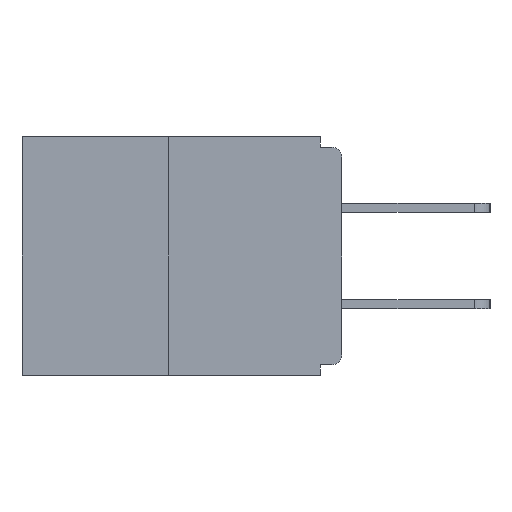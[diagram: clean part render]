
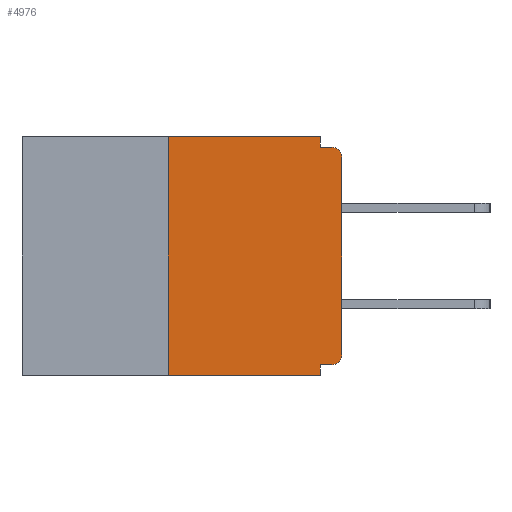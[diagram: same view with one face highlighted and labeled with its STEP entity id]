
A CAD part, left-side view. The second image highlights one B-rep face of the part: STEP entity #4976.
In plain terms, the highlighted planar face has unit normal (-1, 0, 0).
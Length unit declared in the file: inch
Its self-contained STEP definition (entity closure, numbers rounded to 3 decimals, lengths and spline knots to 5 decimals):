
#31 = EDGE_CURVE ( 'NONE', #18143, #26594, #9103, .T. ) ;
#90 = EDGE_CURVE ( 'NONE', #26594, #7525, #13710, .T. ) ;
#605 = AXIS2_PLACEMENT_3D ( 'NONE', #1135, #11697, #5439 ) ;
#971 = LINE ( 'NONE', #27043, #14540 ) ;
#1135 = CARTESIAN_POINT ( 'NONE',  ( 0., 0.015, -0.03 ) ) ;
#1217 = CARTESIAN_POINT ( 'NONE',  ( 0., 0.46, -0.343 ) ) ;
#1404 = ORIENTED_EDGE ( 'NONE', *, *, #26689, .T. ) ;
#2222 = CARTESIAN_POINT ( 'NONE',  ( 0., 0.015, -0.015 ) ) ;
#2550 = EDGE_CURVE ( 'NONE', #18143, #7772, #5038, .T. ) ;
#2584 = DIRECTION ( 'NONE',  ( 0., -1., 0. ) ) ;
#3198 = EDGE_CURVE ( 'NONE', #11646, #19144, #18828, .T. ) ;
#3662 = LINE ( 'NONE', #16313, #14893 ) ;
#3690 = DIRECTION ( 'NONE',  ( 0., 0., 1. ) ) ;
#4295 = CARTESIAN_POINT ( 'NONE',  ( 0., 0.25, -0.343 ) ) ;
#4530 = CARTESIAN_POINT ( 'NONE',  ( 0., 0., -0.03 ) ) ;
#4556 = ORIENTED_EDGE ( 'NONE', *, *, #24536, .T. ) ;
#4976 = ADVANCED_FACE ( 'NONE', ( #19230 ), #17093, .F. ) ;
#5038 = CIRCLE ( 'NONE', #27012, 0.015 ) ;
#5095 = VERTEX_POINT ( 'NONE', #22793 ) ;
#5439 = DIRECTION ( 'NONE',  ( 0., 0., -1. ) ) ;
#5881 = CARTESIAN_POINT ( 'NONE',  ( 0., 0.031, 0. ) ) ;
#6018 = DIRECTION ( 'NONE',  ( 0., 0., 1. ) ) ;
#6752 = LINE ( 'NONE', #5881, #17272 ) ;
#7511 = CIRCLE ( 'NONE', #605, 0.015 ) ;
#7525 = VERTEX_POINT ( 'NONE', #13247 ) ;
#7681 = EDGE_LOOP ( 'NONE', ( #19044, #13883, #1404, #14163, #9592, #15744, #4556, #9803, #15770, #14774 ) ) ;
#7722 = LINE ( 'NONE', #12929, #23861 ) ;
#7772 = VERTEX_POINT ( 'NONE', #14413 ) ;
#7925 = DIRECTION ( 'NONE',  ( 0., 0., -1. ) ) ;
#8393 = CARTESIAN_POINT ( 'NONE',  ( 0., 0.031, -0.343 ) ) ;
#9103 = LINE ( 'NONE', #14466, #15397 ) ;
#9592 = ORIENTED_EDGE ( 'NONE', *, *, #31, .F. ) ;
#9803 = ORIENTED_EDGE ( 'NONE', *, *, #20146, .T. ) ;
#10143 = DIRECTION ( 'NONE',  ( 0., 1., 0. ) ) ;
#11646 = VERTEX_POINT ( 'NONE', #24888 ) ;
#11697 = DIRECTION ( 'NONE',  ( -1., 0., 0. ) ) ;
#12929 = CARTESIAN_POINT ( 'NONE',  ( 0., 0., 0. ) ) ;
#13247 = CARTESIAN_POINT ( 'NONE',  ( 0., 0.031, -0.343 ) ) ;
#13315 = AXIS2_PLACEMENT_3D ( 'NONE', #15324, #21396, #23334 ) ;
#13623 = CARTESIAN_POINT ( 'NONE',  ( 0., 0.25, 0. ) ) ;
#13710 = LINE ( 'NONE', #8393, #18666 ) ;
#13883 = ORIENTED_EDGE ( 'NONE', *, *, #18235, .F. ) ;
#14163 = ORIENTED_EDGE ( 'NONE', *, *, #90, .F. ) ;
#14176 = VECTOR ( 'NONE', #16964, 39.37008 ) ;
#14413 = CARTESIAN_POINT ( 'NONE',  ( 0., 0., -0.313 ) ) ;
#14466 = CARTESIAN_POINT ( 'NONE',  ( 0., 0., -0.328 ) ) ;
#14540 = VECTOR ( 'NONE', #2584, 39.37008 ) ;
#14774 = ORIENTED_EDGE ( 'NONE', *, *, #15347, .F. ) ;
#14893 = VECTOR ( 'NONE', #3690, 39.37008 ) ;
#15324 = CARTESIAN_POINT ( 'NONE',  ( 0., 0.46, 0. ) ) ;
#15347 = EDGE_CURVE ( 'NONE', #5095, #11646, #6752, .T. ) ;
#15397 = VECTOR ( 'NONE', #10143, 39.37008 ) ;
#15744 = ORIENTED_EDGE ( 'NONE', *, *, #2550, .T. ) ;
#15770 = ORIENTED_EDGE ( 'NONE', *, *, #3198, .F. ) ;
#15941 = CARTESIAN_POINT ( 'NONE',  ( 0., 0.015, -0.328 ) ) ;
#16313 = CARTESIAN_POINT ( 'NONE',  ( 0., 0.25, 0. ) ) ;
#16480 = EDGE_CURVE ( 'NONE', #21625, #5095, #971, .T. ) ;
#16964 = DIRECTION ( 'NONE',  ( 0., -1., 0. ) ) ;
#17093 = PLANE ( 'NONE',  #13315 ) ;
#17272 = VECTOR ( 'NONE', #18227, 39.37008 ) ;
#17790 = VECTOR ( 'NONE', #22819, 39.37008 ) ;
#18143 = VERTEX_POINT ( 'NONE', #15941 ) ;
#18227 = DIRECTION ( 'NONE',  ( 0., 0., -1. ) ) ;
#18235 = EDGE_CURVE ( 'NONE', #20836, #21625, #3662, .T. ) ;
#18666 = VECTOR ( 'NONE', #18795, 39.37008 ) ;
#18795 = DIRECTION ( 'NONE',  ( 0., 0., -1. ) ) ;
#18828 = LINE ( 'NONE', #21000, #14176 ) ;
#19044 = ORIENTED_EDGE ( 'NONE', *, *, #16480, .F. ) ;
#19144 = VERTEX_POINT ( 'NONE', #2222 ) ;
#19230 = FACE_OUTER_BOUND ( 'NONE', #7681, .T. ) ;
#19625 = VERTEX_POINT ( 'NONE', #4530 ) ;
#20146 = EDGE_CURVE ( 'NONE', #19625, #19144, #7511, .T. ) ;
#20836 = VERTEX_POINT ( 'NONE', #4295 ) ;
#21000 = CARTESIAN_POINT ( 'NONE',  ( 0., 0., -0.015 ) ) ;
#21396 = DIRECTION ( 'NONE',  ( 1., 0., 0. ) ) ;
#21625 = VERTEX_POINT ( 'NONE', #13623 ) ;
#22665 = CARTESIAN_POINT ( 'NONE',  ( 0., 0.015, -0.313 ) ) ;
#22793 = CARTESIAN_POINT ( 'NONE',  ( 0., 0.031, 0. ) ) ;
#22819 = DIRECTION ( 'NONE',  ( 0., -1., 0. ) ) ;
#23334 = DIRECTION ( 'NONE',  ( 0., 0., -1. ) ) ;
#23861 = VECTOR ( 'NONE', #6018, 39.37008 ) ;
#24536 = EDGE_CURVE ( 'NONE', #7772, #19625, #7722, .T. ) ;
#24868 = DIRECTION ( 'NONE',  ( -1., 0., 0. ) ) ;
#24888 = CARTESIAN_POINT ( 'NONE',  ( 0., 0.031, -0.015 ) ) ;
#25391 = LINE ( 'NONE', #1217, #17790 ) ;
#26050 = CARTESIAN_POINT ( 'NONE',  ( 0., 0.031, -0.328 ) ) ;
#26594 = VERTEX_POINT ( 'NONE', #26050 ) ;
#26689 = EDGE_CURVE ( 'NONE', #20836, #7525, #25391, .T. ) ;
#27012 = AXIS2_PLACEMENT_3D ( 'NONE', #22665, #24868, #7925 ) ;
#27043 = CARTESIAN_POINT ( 'NONE',  ( 0., 0.46, 0. ) ) ;
